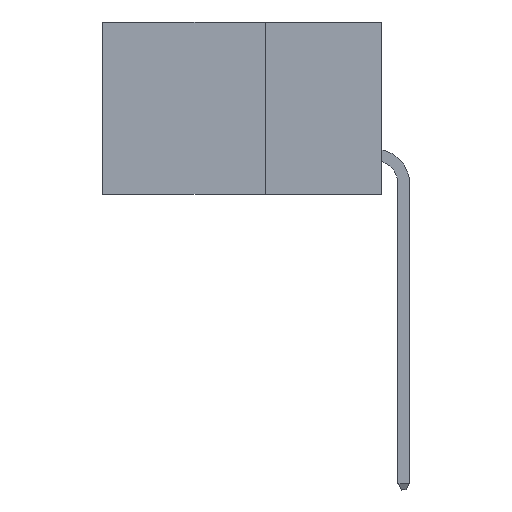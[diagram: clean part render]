
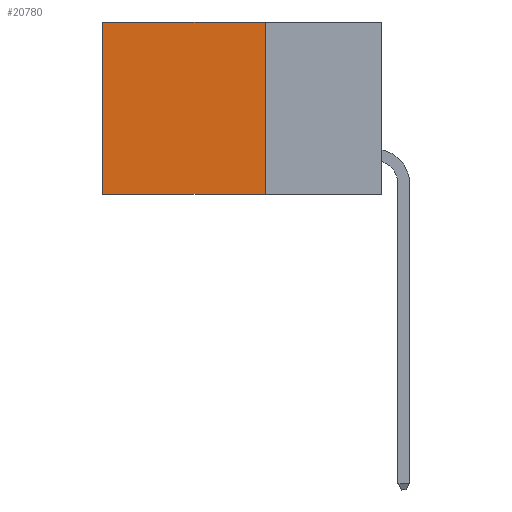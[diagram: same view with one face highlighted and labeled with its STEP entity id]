
A CAD part, left-side view. The second image highlights one B-rep face of the part: STEP entity #20780.
In plain terms, the highlighted planar face has unit normal (-1, 0, 0).
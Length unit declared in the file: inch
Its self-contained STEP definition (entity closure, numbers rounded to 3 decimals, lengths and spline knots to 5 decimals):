
#435 = VERTEX_POINT ( 'NONE', #29235 ) ;
#468 = VECTOR ( 'NONE', #46131, 39.37008 ) ;
#1982 = DIRECTION ( 'NONE',  ( 0., 1., 0. ) ) ;
#2387 = VECTOR ( 'NONE', #1982, 39.37008 ) ;
#2503 = EDGE_CURVE ( 'NONE', #42038, #18842, #28678, .T. ) ;
#5222 = CARTESIAN_POINT ( 'NONE',  ( 0.2875, 0.25, -0.37 ) ) ;
#6323 = PLANE ( 'NONE',  #42776 ) ;
#8153 = EDGE_CURVE ( 'NONE', #16355, #435, #8579, .T. ) ;
#8579 = LINE ( 'NONE', #45285, #2387 ) ;
#8935 = CARTESIAN_POINT ( 'NONE',  ( 0.2875, 0.25, -0.37 ) ) ;
#9954 = CARTESIAN_POINT ( 'NONE',  ( 0.2875, 0.25, 0. ) ) ;
#10665 = CARTESIAN_POINT ( 'NONE',  ( 0.2875, 0.25, 0. ) ) ;
#12540 = VECTOR ( 'NONE', #44632, 39.37008 ) ;
#15791 = VECTOR ( 'NONE', #37942, 39.37008 ) ;
#15804 = EDGE_CURVE ( 'NONE', #16355, #42038, #19521, .T. ) ;
#16355 = VERTEX_POINT ( 'NONE', #30363 ) ;
#16749 = EDGE_LOOP ( 'NONE', ( #33916, #31483, #45632, #18562 ) ) ;
#17142 = DIRECTION ( 'NONE',  ( 1., 0., 0. ) ) ;
#18562 = ORIENTED_EDGE ( 'NONE', *, *, #8153, .T. ) ;
#18842 = VERTEX_POINT ( 'NONE', #31003 ) ;
#19521 = LINE ( 'NONE', #10665, #468 ) ;
#20780 = ADVANCED_FACE ( 'NONE', ( #42034 ), #6323, .F. ) ;
#24621 = DIRECTION ( 'NONE',  ( 0., 0., -1. ) ) ;
#28678 = LINE ( 'NONE', #5222, #15791 ) ;
#29235 = CARTESIAN_POINT ( 'NONE',  ( 0.2875, 0.6, 0. ) ) ;
#30363 = CARTESIAN_POINT ( 'NONE',  ( 0.2875, 0.25, 0. ) ) ;
#31003 = CARTESIAN_POINT ( 'NONE',  ( 0.2875, 0.6, -0.37 ) ) ;
#31483 = ORIENTED_EDGE ( 'NONE', *, *, #2503, .F. ) ;
#33916 = ORIENTED_EDGE ( 'NONE', *, *, #45798, .T. ) ;
#37942 = DIRECTION ( 'NONE',  ( 0., 1., 0. ) ) ;
#41125 = CARTESIAN_POINT ( 'NONE',  ( 0.2875, 0.6, 0. ) ) ;
#42034 = FACE_OUTER_BOUND ( 'NONE', #16749, .T. ) ;
#42038 = VERTEX_POINT ( 'NONE', #8935 ) ;
#42253 = LINE ( 'NONE', #41125, #12540 ) ;
#42776 = AXIS2_PLACEMENT_3D ( 'NONE', #9954, #17142, #24621 ) ;
#44632 = DIRECTION ( 'NONE',  ( 0., 0., -1. ) ) ;
#45285 = CARTESIAN_POINT ( 'NONE',  ( 0.2875, 0.25, 0. ) ) ;
#45632 = ORIENTED_EDGE ( 'NONE', *, *, #15804, .F. ) ;
#45798 = EDGE_CURVE ( 'NONE', #435, #18842, #42253, .T. ) ;
#46131 = DIRECTION ( 'NONE',  ( 0., 0., -1. ) ) ;
